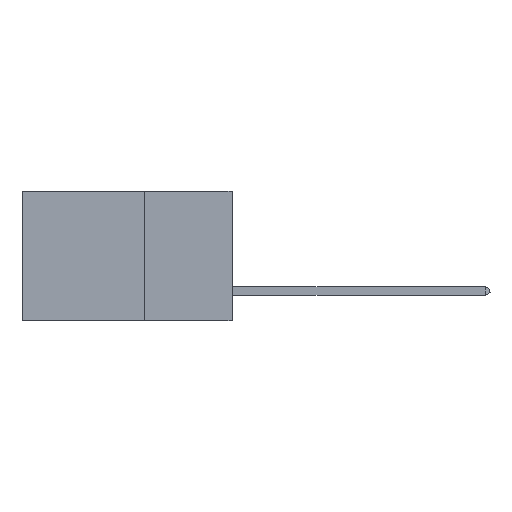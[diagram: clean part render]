
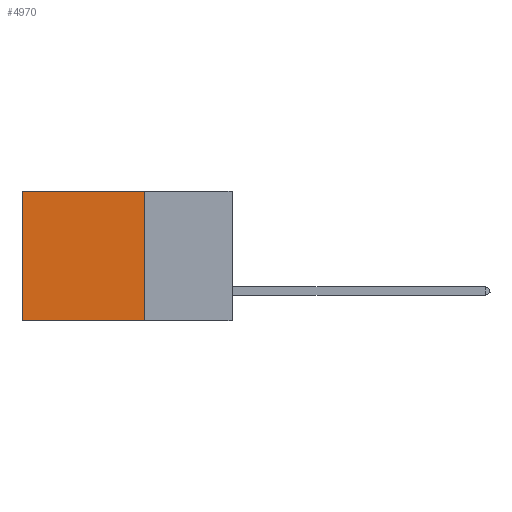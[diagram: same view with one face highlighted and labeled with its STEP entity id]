
A CAD part, left-side view. The second image highlights one B-rep face of the part: STEP entity #4970.
In plain terms, the highlighted planar face has unit normal (-1, 0, 0).
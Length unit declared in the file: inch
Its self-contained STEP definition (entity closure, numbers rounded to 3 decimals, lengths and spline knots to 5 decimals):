
#593 = CARTESIAN_POINT ( 'NONE',  ( 0.2875, 0.25, 0. ) ) ;
#654 = CARTESIAN_POINT ( 'NONE',  ( 0.2875, 0.25, 0. ) ) ;
#1562 = ORIENTED_EDGE ( 'NONE', *, *, #28129, .T. ) ;
#2395 = ORIENTED_EDGE ( 'NONE', *, *, #12498, .F. ) ;
#2534 = VERTEX_POINT ( 'NONE', #25563 ) ;
#4970 = ADVANCED_FACE ( 'NONE', ( #38859 ), #14737, .F. ) ;
#7914 = DIRECTION ( 'NONE',  ( 0., 0., -1. ) ) ;
#10832 = VECTOR ( 'NONE', #33783, 39.37008 ) ;
#11145 = LINE ( 'NONE', #36847, #25671 ) ;
#12498 = EDGE_CURVE ( 'NONE', #36785, #21888, #20828, .T. ) ;
#14737 = PLANE ( 'NONE',  #43751 ) ;
#15032 = DIRECTION ( 'NONE',  ( 0., 0., -1. ) ) ;
#16145 = LINE ( 'NONE', #33537, #31838 ) ;
#16161 = VECTOR ( 'NONE', #20854, 39.37008 ) ;
#18239 = CARTESIAN_POINT ( 'NONE',  ( 0.2875, 0.6, 0. ) ) ;
#18956 = CARTESIAN_POINT ( 'NONE',  ( 0.2875, 0.25, 0. ) ) ;
#20216 = CARTESIAN_POINT ( 'NONE',  ( 0.2875, 0.25, 0. ) ) ;
#20828 = LINE ( 'NONE', #20216, #16161 ) ;
#20854 = DIRECTION ( 'NONE',  ( 0., 0., -1. ) ) ;
#21888 = VERTEX_POINT ( 'NONE', #43547 ) ;
#23007 = ORIENTED_EDGE ( 'NONE', *, *, #34246, .F. ) ;
#23643 = VERTEX_POINT ( 'NONE', #18239 ) ;
#25563 = CARTESIAN_POINT ( 'NONE',  ( 0.2875, 0.6, -0.37 ) ) ;
#25671 = VECTOR ( 'NONE', #41118, 39.37008 ) ;
#26872 = ORIENTED_EDGE ( 'NONE', *, *, #39809, .T. ) ;
#28129 = EDGE_CURVE ( 'NONE', #23643, #2534, #16145, .T. ) ;
#30148 = DIRECTION ( 'NONE',  ( 1., 0., 0. ) ) ;
#31838 = VECTOR ( 'NONE', #15032, 39.37008 ) ;
#33537 = CARTESIAN_POINT ( 'NONE',  ( 0.2875, 0.6, 0. ) ) ;
#33783 = DIRECTION ( 'NONE',  ( 0., 1., 0. ) ) ;
#34246 = EDGE_CURVE ( 'NONE', #21888, #2534, #11145, .T. ) ;
#36785 = VERTEX_POINT ( 'NONE', #654 ) ;
#36847 = CARTESIAN_POINT ( 'NONE',  ( 0.2875, 0.25, -0.37 ) ) ;
#38859 = FACE_OUTER_BOUND ( 'NONE', #46633, .T. ) ;
#39809 = EDGE_CURVE ( 'NONE', #36785, #23643, #44542, .T. ) ;
#41118 = DIRECTION ( 'NONE',  ( 0., 1., 0. ) ) ;
#43547 = CARTESIAN_POINT ( 'NONE',  ( 0.2875, 0.25, -0.37 ) ) ;
#43751 = AXIS2_PLACEMENT_3D ( 'NONE', #18956, #30148, #7914 ) ;
#44542 = LINE ( 'NONE', #593, #10832 ) ;
#46633 = EDGE_LOOP ( 'NONE', ( #1562, #23007, #2395, #26872 ) ) ;
